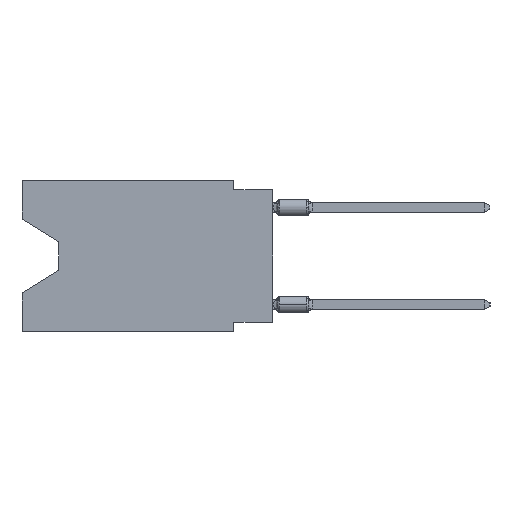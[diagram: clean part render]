
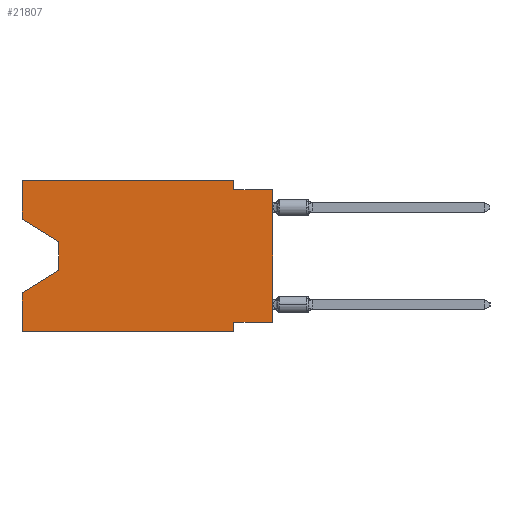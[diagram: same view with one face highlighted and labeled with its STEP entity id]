
A CAD part, left-side view. The second image highlights one B-rep face of the part: STEP entity #21807.
In plain terms, the highlighted planar face has unit normal (-1, 0, 0).
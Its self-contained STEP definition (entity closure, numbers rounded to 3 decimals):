
#282 = DIRECTION ( 'NONE',  ( 0., 0., -1. ) ) ;
#864 = CARTESIAN_POINT ( 'NONE',  ( 0., 16.383, -9.906 ) ) ;
#914 = CARTESIAN_POINT ( 'NONE',  ( 0., 0., -0.635 ) ) ;
#1042 = EDGE_CURVE ( 'NONE', #16375, #5497, #37423, .T. ) ;
#1156 = LINE ( 'NONE', #13100, #19492 ) ;
#1512 = LINE ( 'NONE', #22178, #9371 ) ;
#1702 = EDGE_CURVE ( 'NONE', #15532, #11189, #16572, .T. ) ;
#2026 = VERTEX_POINT ( 'NONE', #15763 ) ;
#2236 = ORIENTED_EDGE ( 'NONE', *, *, #9464, .T. ) ;
#2961 = EDGE_CURVE ( 'NONE', #16375, #15532, #32843, .T. ) ;
#3240 = CARTESIAN_POINT ( 'NONE',  ( 0., 0., -0.635 ) ) ;
#3561 = ORIENTED_EDGE ( 'NONE', *, *, #8095, .F. ) ;
#3783 = ORIENTED_EDGE ( 'NONE', *, *, #6028, .T. ) ;
#4561 = CARTESIAN_POINT ( 'NONE',  ( 0., 16.383, -2.546 ) ) ;
#5497 = VERTEX_POINT ( 'NONE', #15283 ) ;
#5793 = ORIENTED_EDGE ( 'NONE', *, *, #20204, .F. ) ;
#6028 = EDGE_CURVE ( 'NONE', #5497, #31784, #1512, .T. ) ;
#6613 = DIRECTION ( 'NONE',  ( 0., 0., -1. ) ) ;
#6813 = DIRECTION ( 'NONE',  ( 0., 0.855, -0.519 ) ) ;
#6837 = DIRECTION ( 'NONE',  ( 1., 0., 0. ) ) ;
#6843 = DIRECTION ( 'NONE',  ( 0., -1., 0. ) ) ;
#7826 = EDGE_LOOP ( 'NONE', ( #13634, #3783, #20453, #24128, #10336, #23313, #5793, #2236, #21979, #3561, #26737, #31125 ) ) ;
#7958 = PLANE ( 'NONE',  #10076 ) ;
#8095 = EDGE_CURVE ( 'NONE', #11189, #2026, #9154, .T. ) ;
#9154 = LINE ( 'NONE', #11836, #12440 ) ;
#9371 = VECTOR ( 'NONE', #27418, 1000. ) ;
#9464 = EDGE_CURVE ( 'NONE', #29021, #18696, #13638, .T. ) ;
#9600 = VERTEX_POINT ( 'NONE', #38023 ) ;
#10076 = AXIS2_PLACEMENT_3D ( 'NONE', #19727, #6837, #282 ) ;
#10336 = ORIENTED_EDGE ( 'NONE', *, *, #28254, .T. ) ;
#10566 = DIRECTION ( 'NONE',  ( 0., 0., 1. ) ) ;
#11189 = VERTEX_POINT ( 'NONE', #23404 ) ;
#11252 = CARTESIAN_POINT ( 'NONE',  ( 0., 0., -9.271 ) ) ;
#11836 = CARTESIAN_POINT ( 'NONE',  ( 0., 2.54, 0. ) ) ;
#12440 = VECTOR ( 'NONE', #36230, 1000. ) ;
#12904 = VECTOR ( 'NONE', #28128, 1000. ) ;
#13100 = CARTESIAN_POINT ( 'NONE',  ( 0., 16.383, 0. ) ) ;
#13634 = ORIENTED_EDGE ( 'NONE', *, *, #1042, .T. ) ;
#13638 = LINE ( 'NONE', #15974, #27880 ) ;
#14456 = CARTESIAN_POINT ( 'NONE',  ( 0., 13.97, -5.893 ) ) ;
#14477 = VECTOR ( 'NONE', #18289, 1000. ) ;
#15202 = CARTESIAN_POINT ( 'NONE',  ( 0., 16.383, -2.546 ) ) ;
#15283 = CARTESIAN_POINT ( 'NONE',  ( 0., 13.97, -4.013 ) ) ;
#15517 = LINE ( 'NONE', #864, #25496 ) ;
#15532 = VERTEX_POINT ( 'NONE', #22844 ) ;
#15763 = CARTESIAN_POINT ( 'NONE',  ( 0., 2.54, -0.635 ) ) ;
#15974 = CARTESIAN_POINT ( 'NONE',  ( 0., 0., 0. ) ) ;
#16375 = VERTEX_POINT ( 'NONE', #15202 ) ;
#16567 = CARTESIAN_POINT ( 'NONE',  ( 0., 2.54, -9.906 ) ) ;
#16572 = LINE ( 'NONE', #37663, #27900 ) ;
#16866 = VECTOR ( 'NONE', #36502, 1000. ) ;
#17339 = DIRECTION ( 'NONE',  ( 0., -1., 0. ) ) ;
#17704 = EDGE_CURVE ( 'NONE', #24082, #9600, #1156, .T. ) ;
#18289 = DIRECTION ( 'NONE',  ( 0., -1., 0. ) ) ;
#18696 = VERTEX_POINT ( 'NONE', #3240 ) ;
#19492 = VECTOR ( 'NONE', #32877, 1000. ) ;
#19727 = CARTESIAN_POINT ( 'NONE',  ( 0., 16.383, 0. ) ) ;
#20151 = DIRECTION ( 'NONE',  ( 0., 1., 0. ) ) ;
#20204 = EDGE_CURVE ( 'NONE', #29021, #33655, #25768, .T. ) ;
#20412 = EDGE_CURVE ( 'NONE', #33655, #24739, #23809, .T. ) ;
#20453 = ORIENTED_EDGE ( 'NONE', *, *, #31270, .T. ) ;
#21091 = CARTESIAN_POINT ( 'NONE',  ( 0., 16.383, -9.906 ) ) ;
#21493 = CARTESIAN_POINT ( 'NONE',  ( 0., 13.97, -5.893 ) ) ;
#21807 = ADVANCED_FACE ( 'NONE', ( #25535 ), #7958, .F. ) ;
#21979 = ORIENTED_EDGE ( 'NONE', *, *, #23527, .F. ) ;
#22178 = CARTESIAN_POINT ( 'NONE',  ( 0., 13.97, -4.013 ) ) ;
#22844 = CARTESIAN_POINT ( 'NONE',  ( 0., 16.383, 0. ) ) ;
#23313 = ORIENTED_EDGE ( 'NONE', *, *, #20412, .F. ) ;
#23404 = CARTESIAN_POINT ( 'NONE',  ( 0., 2.54, 0. ) ) ;
#23527 = EDGE_CURVE ( 'NONE', #2026, #18696, #27939, .T. ) ;
#23809 = LINE ( 'NONE', #35631, #34241 ) ;
#24082 = VERTEX_POINT ( 'NONE', #21091 ) ;
#24128 = ORIENTED_EDGE ( 'NONE', *, *, #17704, .F. ) ;
#24712 = VECTOR ( 'NONE', #6813, 1000. ) ;
#24739 = VERTEX_POINT ( 'NONE', #16567 ) ;
#25496 = VECTOR ( 'NONE', #6843, 1000. ) ;
#25535 = FACE_OUTER_BOUND ( 'NONE', #7826, .T. ) ;
#25768 = LINE ( 'NONE', #11252, #29845 ) ;
#26737 = ORIENTED_EDGE ( 'NONE', *, *, #1702, .F. ) ;
#27417 = CARTESIAN_POINT ( 'NONE',  ( 0., 16.383, 0. ) ) ;
#27418 = DIRECTION ( 'NONE',  ( 0., 0., -1. ) ) ;
#27880 = VECTOR ( 'NONE', #10566, 1000. ) ;
#27900 = VECTOR ( 'NONE', #17339, 1000. ) ;
#27939 = LINE ( 'NONE', #914, #14477 ) ;
#28128 = DIRECTION ( 'NONE',  ( 0., -0.855, -0.519 ) ) ;
#28254 = EDGE_CURVE ( 'NONE', #24082, #24739, #15517, .T. ) ;
#29021 = VERTEX_POINT ( 'NONE', #32864 ) ;
#29845 = VECTOR ( 'NONE', #20151, 1000. ) ;
#31125 = ORIENTED_EDGE ( 'NONE', *, *, #2961, .F. ) ;
#31218 = CARTESIAN_POINT ( 'NONE',  ( 0., 2.54, -9.271 ) ) ;
#31270 = EDGE_CURVE ( 'NONE', #31784, #9600, #32921, .T. ) ;
#31784 = VERTEX_POINT ( 'NONE', #14456 ) ;
#32843 = LINE ( 'NONE', #27417, #16866 ) ;
#32864 = CARTESIAN_POINT ( 'NONE',  ( 0., 0., -9.271 ) ) ;
#32877 = DIRECTION ( 'NONE',  ( 0., 0., 1. ) ) ;
#32921 = LINE ( 'NONE', #21493, #24712 ) ;
#33655 = VERTEX_POINT ( 'NONE', #31218 ) ;
#34241 = VECTOR ( 'NONE', #6613, 1000. ) ;
#35631 = CARTESIAN_POINT ( 'NONE',  ( 0., 2.54, -9.906 ) ) ;
#36230 = DIRECTION ( 'NONE',  ( 0., 0., -1. ) ) ;
#36502 = DIRECTION ( 'NONE',  ( 0., 0., 1. ) ) ;
#37423 = LINE ( 'NONE', #4561, #12904 ) ;
#37663 = CARTESIAN_POINT ( 'NONE',  ( 0., 16.383, 0. ) ) ;
#38023 = CARTESIAN_POINT ( 'NONE',  ( 0., 16.383, -7.36 ) ) ;
